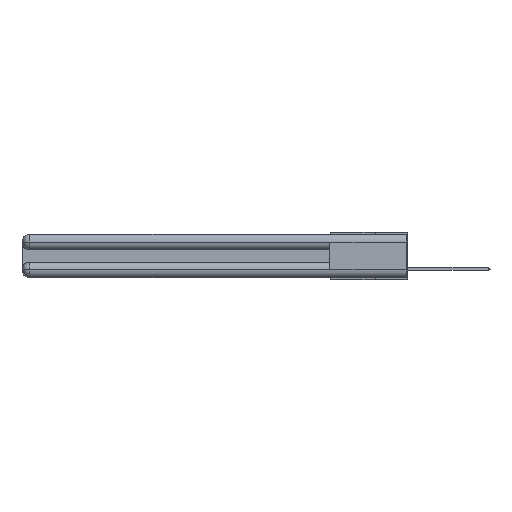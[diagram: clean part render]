
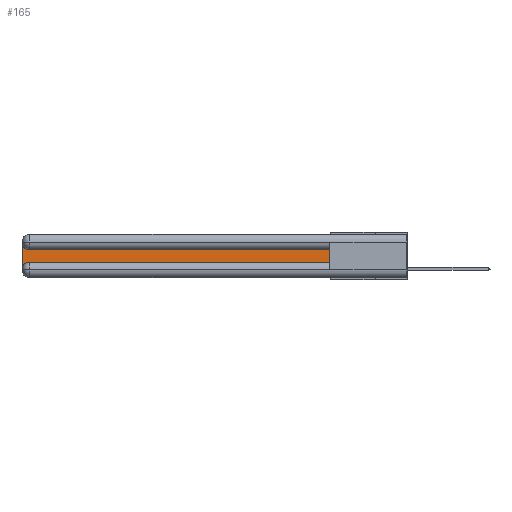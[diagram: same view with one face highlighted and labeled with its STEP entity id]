
A CAD part, left-side view. The second image highlights one B-rep face of the part: STEP entity #165.
In plain terms, the highlighted planar face has unit normal (-1, 0, 0).
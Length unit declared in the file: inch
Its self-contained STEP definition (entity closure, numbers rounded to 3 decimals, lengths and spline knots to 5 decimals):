
#165 = ADVANCED_FACE ( 'NONE', ( #4914 ), #21588, .F. ) ;
#665 = VECTOR ( 'NONE', #14165, 39.37008 ) ;
#884 = ORIENTED_EDGE ( 'NONE', *, *, #19510, .T. ) ;
#3105 = CARTESIAN_POINT ( 'NONE',  ( 0.075, 2.94, -0.2175 ) ) ;
#3722 = DIRECTION ( 'NONE',  ( 0., 1., 0. ) ) ;
#3965 = CARTESIAN_POINT ( 'NONE',  ( 0.075, 0.6, -0.2175 ) ) ;
#4914 = FACE_OUTER_BOUND ( 'NONE', #10083, .T. ) ;
#5159 = ORIENTED_EDGE ( 'NONE', *, *, #12699, .T. ) ;
#5606 = CARTESIAN_POINT ( 'NONE',  ( 0.075, 0.6, -0.1225 ) ) ;
#6015 = LINE ( 'NONE', #10029, #11341 ) ;
#7186 = DIRECTION ( 'NONE',  ( 0., 0., -1. ) ) ;
#7579 = AXIS2_PLACEMENT_3D ( 'NONE', #18791, #13871, #19030 ) ;
#8895 = CARTESIAN_POINT ( 'NONE',  ( 0.075, 0.6, -0.1225 ) ) ;
#9140 = DIRECTION ( 'NONE',  ( 0., 0., 1. ) ) ;
#9823 = ORIENTED_EDGE ( 'NONE', *, *, #29964, .T. ) ;
#10029 = CARTESIAN_POINT ( 'NONE',  ( 0.075, 3., -0.2175 ) ) ;
#10083 = EDGE_LOOP ( 'NONE', ( #31302, #24561, #9823, #17573, #884, #5159 ) ) ;
#10810 = EDGE_CURVE ( 'NONE', #25361, #19288, #14521, .T. ) ;
#11341 = VECTOR ( 'NONE', #28339, 39.37008 ) ;
#12023 = EDGE_CURVE ( 'NONE', #31681, #25361, #12082, .T. ) ;
#12082 = LINE ( 'NONE', #8895, #20205 ) ;
#12699 = EDGE_CURVE ( 'NONE', #14325, #31681, #27077, .T. ) ;
#13871 = DIRECTION ( 'NONE',  ( 1., 0., 0. ) ) ;
#14165 = DIRECTION ( 'NONE',  ( 0., -1., 0. ) ) ;
#14325 = VERTEX_POINT ( 'NONE', #21247 ) ;
#14521 = CIRCLE ( 'NONE', #7579, 0.06 ) ;
#16067 = VECTOR ( 'NONE', #9140, 39.37008 ) ;
#16110 = DIRECTION ( 'NONE',  ( 0., 0., -1. ) ) ;
#17537 = DIRECTION ( 'NONE',  ( 1., 0., 0. ) ) ;
#17573 = ORIENTED_EDGE ( 'NONE', *, *, #18093, .T. ) ;
#18093 = EDGE_CURVE ( 'NONE', #32442, #22809, #20831, .T. ) ;
#18791 = CARTESIAN_POINT ( 'NONE',  ( 0.075, 2.94, -0.0625 ) ) ;
#19030 = DIRECTION ( 'NONE',  ( 0., 0., -1. ) ) ;
#19288 = VERTEX_POINT ( 'NONE', #23386 ) ;
#19510 = EDGE_CURVE ( 'NONE', #22809, #14325, #33366, .T. ) ;
#20156 = CARTESIAN_POINT ( 'NONE',  ( 0.075, 2.94, -0.2775 ) ) ;
#20205 = VECTOR ( 'NONE', #3722, 39.37008 ) ;
#20831 = CIRCLE ( 'NONE', #25145, 0.06 ) ;
#21247 = CARTESIAN_POINT ( 'NONE',  ( 0.075, 0.6, -0.2175 ) ) ;
#21588 = PLANE ( 'NONE',  #27608 ) ;
#21930 = CARTESIAN_POINT ( 'NONE',  ( 0.075, 0.6, -0.2175 ) ) ;
#22809 = VERTEX_POINT ( 'NONE', #3105 ) ;
#23386 = CARTESIAN_POINT ( 'NONE',  ( 0.075, 3., -0.0625 ) ) ;
#24178 = CARTESIAN_POINT ( 'NONE',  ( 0.075, 3., -0.1225 ) ) ;
#24561 = ORIENTED_EDGE ( 'NONE', *, *, #10810, .T. ) ;
#25145 = AXIS2_PLACEMENT_3D ( 'NONE', #20156, #17537, #7186 ) ;
#25361 = VERTEX_POINT ( 'NONE', #28858 ) ;
#25370 = CARTESIAN_POINT ( 'NONE',  ( 0.075, 3., -0.2775 ) ) ;
#27077 = LINE ( 'NONE', #3965, #16067 ) ;
#27608 = AXIS2_PLACEMENT_3D ( 'NONE', #24178, #29078, #16110 ) ;
#28339 = DIRECTION ( 'NONE',  ( 0., 0., -1. ) ) ;
#28858 = CARTESIAN_POINT ( 'NONE',  ( 0.075, 2.94, -0.1225 ) ) ;
#29078 = DIRECTION ( 'NONE',  ( 1., 0., 0. ) ) ;
#29964 = EDGE_CURVE ( 'NONE', #19288, #32442, #6015, .T. ) ;
#31302 = ORIENTED_EDGE ( 'NONE', *, *, #12023, .T. ) ;
#31681 = VERTEX_POINT ( 'NONE', #5606 ) ;
#32442 = VERTEX_POINT ( 'NONE', #25370 ) ;
#33366 = LINE ( 'NONE', #21930, #665 ) ;
